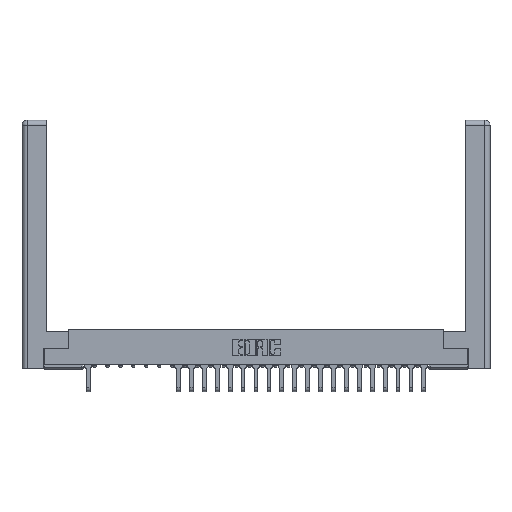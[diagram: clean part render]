
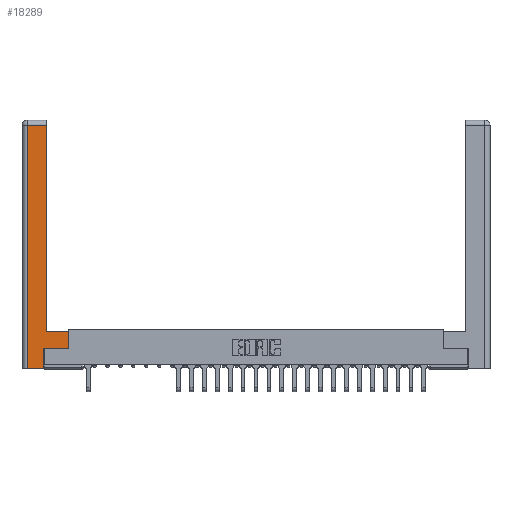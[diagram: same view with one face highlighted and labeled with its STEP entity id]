
A CAD part, top view. The second image highlights one B-rep face of the part: STEP entity #18289.
In plain terms, the highlighted planar face has unit normal (0, 0, 1).
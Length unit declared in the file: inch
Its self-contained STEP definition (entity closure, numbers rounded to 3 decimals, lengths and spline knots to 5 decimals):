
#552 = EDGE_CURVE ( 'NONE', #20814, #8181, #4727, .T. ) ;
#794 = ORIENTED_EDGE ( 'NONE', *, *, #2090, .T. ) ;
#911 = LINE ( 'NONE', #24235, #12553 ) ;
#917 = CARTESIAN_POINT ( 'NONE',  ( 0.295, 2.94, 0. ) ) ;
#1099 = ORIENTED_EDGE ( 'NONE', *, *, #15657, .T. ) ;
#1510 = CARTESIAN_POINT ( 'NONE',  ( 0.0615, 0., 0. ) ) ;
#1676 = EDGE_CURVE ( 'NONE', #12313, #20814, #5750, .T. ) ;
#1831 = ORIENTED_EDGE ( 'NONE', *, *, #552, .T. ) ;
#2090 = EDGE_CURVE ( 'NONE', #28071, #24206, #911, .T. ) ;
#2204 = DIRECTION ( 'NONE',  ( 0., 1., 0. ) ) ;
#2688 = VERTEX_POINT ( 'NONE', #28554 ) ;
#3421 = VECTOR ( 'NONE', #24378, 39.37008 ) ;
#4164 = DIRECTION ( 'NONE',  ( 0., -1., 0. ) ) ;
#4596 = CARTESIAN_POINT ( 'NONE',  ( 0.265, 0.245, 0. ) ) ;
#4651 = ORIENTED_EDGE ( 'NONE', *, *, #1676, .T. ) ;
#4727 = LINE ( 'NONE', #4596, #21502 ) ;
#5230 = LINE ( 'NONE', #27182, #28573 ) ;
#5750 = LINE ( 'NONE', #20620, #17932 ) ;
#6121 = VERTEX_POINT ( 'NONE', #917 ) ;
#6960 = EDGE_CURVE ( 'NONE', #2688, #6121, #15696, .T. ) ;
#8181 = VERTEX_POINT ( 'NONE', #13169 ) ;
#9206 = CARTESIAN_POINT ( 'NONE',  ( 0.265, 0., 0. ) ) ;
#9901 = EDGE_LOOP ( 'NONE', ( #28199, #12581, #25241, #4651, #1831, #1099, #794, #20352 ) ) ;
#10073 = CARTESIAN_POINT ( 'NONE',  ( 0.565, 0.245, 0. ) ) ;
#10216 = LINE ( 'NONE', #29349, #10951 ) ;
#10639 = DIRECTION ( 'NONE',  ( 0., 0., -1. ) ) ;
#10715 = DIRECTION ( 'NONE',  ( 0., 1., 0. ) ) ;
#10951 = VECTOR ( 'NONE', #18260, 39.37008 ) ;
#11087 = CARTESIAN_POINT ( 'NONE',  ( 0.565, 0.245, 0. ) ) ;
#11164 = EDGE_CURVE ( 'NONE', #17409, #12313, #29497, .T. ) ;
#12313 = VERTEX_POINT ( 'NONE', #1510 ) ;
#12368 = DIRECTION ( 'NONE',  ( 1., 0., 0. ) ) ;
#12553 = VECTOR ( 'NONE', #10715, 39.37008 ) ;
#12581 = ORIENTED_EDGE ( 'NONE', *, *, #16091, .T. ) ;
#13169 = CARTESIAN_POINT ( 'NONE',  ( 0.265, 0.245, 0. ) ) ;
#13840 = VECTOR ( 'NONE', #12368, 39.37008 ) ;
#14064 = FACE_OUTER_BOUND ( 'NONE', #9901, .T. ) ;
#14249 = CARTESIAN_POINT ( 'NONE',  ( 0.0615, 2.94, 0. ) ) ;
#14565 = LINE ( 'NONE', #10073, #13840 ) ;
#15657 = EDGE_CURVE ( 'NONE', #8181, #28071, #14565, .T. ) ;
#15696 = LINE ( 'NONE', #26507, #3421 ) ;
#16091 = EDGE_CURVE ( 'NONE', #6121, #17409, #5230, .T. ) ;
#17234 = EDGE_CURVE ( 'NONE', #24206, #2688, #10216, .T. ) ;
#17409 = VERTEX_POINT ( 'NONE', #14249 ) ;
#17932 = VECTOR ( 'NONE', #22795, 39.37008 ) ;
#18260 = DIRECTION ( 'NONE',  ( -1., 0., 0. ) ) ;
#18289 = ADVANCED_FACE ( 'NONE', ( #14064 ), #24164, .F. ) ;
#19551 = CARTESIAN_POINT ( 'NONE',  ( 0., 0., 0. ) ) ;
#20352 = ORIENTED_EDGE ( 'NONE', *, *, #17234, .T. ) ;
#20620 = CARTESIAN_POINT ( 'NONE',  ( 0.265, 0., 0. ) ) ;
#20814 = VERTEX_POINT ( 'NONE', #9206 ) ;
#21502 = VECTOR ( 'NONE', #2204, 39.37008 ) ;
#21814 = CARTESIAN_POINT ( 'NONE',  ( 0.565, 0.45, 0. ) ) ;
#22628 = DIRECTION ( 'NONE',  ( -1., 0., 0. ) ) ;
#22795 = DIRECTION ( 'NONE',  ( 1., 0., 0. ) ) ;
#23605 = VECTOR ( 'NONE', #4164, 39.37008 ) ;
#24164 = PLANE ( 'NONE',  #24946 ) ;
#24206 = VERTEX_POINT ( 'NONE', #21814 ) ;
#24235 = CARTESIAN_POINT ( 'NONE',  ( 0.565, 0.45, 0. ) ) ;
#24378 = DIRECTION ( 'NONE',  ( 0., 1., 0. ) ) ;
#24946 = AXIS2_PLACEMENT_3D ( 'NONE', #19551, #10639, #26405 ) ;
#25241 = ORIENTED_EDGE ( 'NONE', *, *, #11164, .T. ) ;
#26405 = DIRECTION ( 'NONE',  ( -1., 0., 0. ) ) ;
#26507 = CARTESIAN_POINT ( 'NONE',  ( 0.295, 3., 0. ) ) ;
#26806 = CARTESIAN_POINT ( 'NONE',  ( 0.0615, 0., 0. ) ) ;
#27182 = CARTESIAN_POINT ( 'NONE',  ( 0.0615, 2.94, 0. ) ) ;
#28071 = VERTEX_POINT ( 'NONE', #11087 ) ;
#28199 = ORIENTED_EDGE ( 'NONE', *, *, #6960, .T. ) ;
#28554 = CARTESIAN_POINT ( 'NONE',  ( 0.295, 0.45, 0. ) ) ;
#28573 = VECTOR ( 'NONE', #22628, 39.37008 ) ;
#29349 = CARTESIAN_POINT ( 'NONE',  ( 0.295, 0.45, 0. ) ) ;
#29497 = LINE ( 'NONE', #26806, #23605 ) ;
